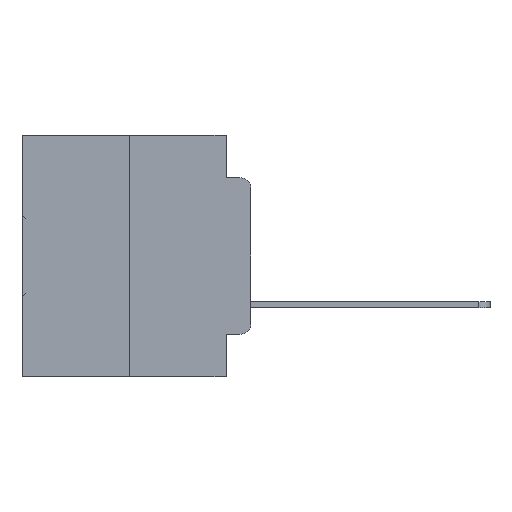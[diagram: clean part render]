
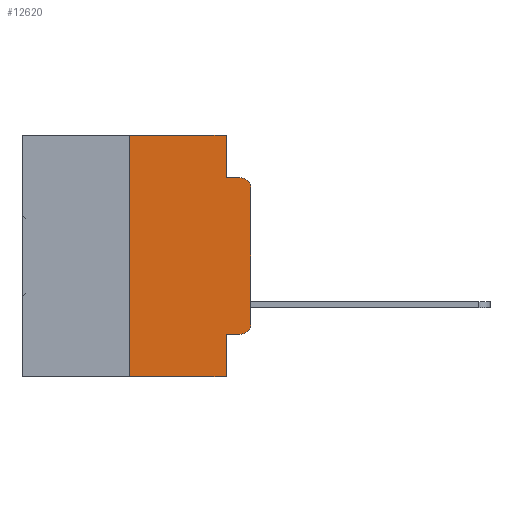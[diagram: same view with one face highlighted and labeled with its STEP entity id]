
A CAD part, left-side view. The second image highlights one B-rep face of the part: STEP entity #12620.
In plain terms, the highlighted planar face has unit normal (-1, 0, 0).
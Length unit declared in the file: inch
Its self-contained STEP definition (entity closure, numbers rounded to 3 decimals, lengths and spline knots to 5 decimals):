
#123 = AXIS2_PLACEMENT_3D ( 'NONE', #13753, #32018, #16451 ) ;
#330 = EDGE_CURVE ( 'NONE', #13568, #7716, #26120, .T. ) ;
#489 = ORIENTED_EDGE ( 'NONE', *, *, #15348, .F. ) ;
#678 = VERTEX_POINT ( 'NONE', #3235 ) ;
#837 = VECTOR ( 'NONE', #24182, 39.37008 ) ;
#2509 = VERTEX_POINT ( 'NONE', #14223 ) ;
#3235 = CARTESIAN_POINT ( 'NONE',  ( 0., 0.02, -0.0885 ) ) ;
#3309 = DIRECTION ( 'NONE',  ( 1., 0., 0. ) ) ;
#3755 = VECTOR ( 'NONE', #12663, 39.37008 ) ;
#3815 = DIRECTION ( 'NONE',  ( 0., 0., -1. ) ) ;
#3931 = CARTESIAN_POINT ( 'NONE',  ( 0., 0., -0.1085 ) ) ;
#4280 = CARTESIAN_POINT ( 'NONE',  ( 0., 0.051, -0.4115 ) ) ;
#6163 = VECTOR ( 'NONE', #3815, 39.37008 ) ;
#6385 = DIRECTION ( 'NONE',  ( 0., 0., -1. ) ) ;
#7286 = LINE ( 'NONE', #34816, #26885 ) ;
#7716 = VERTEX_POINT ( 'NONE', #9987 ) ;
#8122 = EDGE_CURVE ( 'NONE', #13568, #2509, #28965, .T. ) ;
#8532 = LINE ( 'NONE', #21666, #837 ) ;
#8862 = CIRCLE ( 'NONE', #123, 0.02 ) ;
#8866 = CARTESIAN_POINT ( 'NONE',  ( 0., 0.02, -0.1085 ) ) ;
#9408 = CARTESIAN_POINT ( 'NONE',  ( 0., 0.051, 0. ) ) ;
#9987 = CARTESIAN_POINT ( 'NONE',  ( 0., 0.02, -0.4115 ) ) ;
#10120 = VECTOR ( 'NONE', #23786, 39.37008 ) ;
#10635 = VECTOR ( 'NONE', #21236, 39.37008 ) ;
#10929 = ORIENTED_EDGE ( 'NONE', *, *, #330, .T. ) ;
#11174 = PLANE ( 'NONE',  #26160 ) ;
#11584 = DIRECTION ( 'NONE',  ( 0., 0., -1. ) ) ;
#11764 = EDGE_CURVE ( 'NONE', #28743, #16335, #8532, .T. ) ;
#12225 = CARTESIAN_POINT ( 'NONE',  ( 0., 0.051, 0. ) ) ;
#12292 = LINE ( 'NONE', #26441, #10635 ) ;
#12463 = EDGE_CURVE ( 'NONE', #16335, #32840, #12292, .T. ) ;
#12570 = VERTEX_POINT ( 'NONE', #13633 ) ;
#12620 = ADVANCED_FACE ( 'NONE', ( #28355 ), #11174, .F. ) ;
#12636 = CARTESIAN_POINT ( 'NONE',  ( 0., 0.25, 0. ) ) ;
#12663 = DIRECTION ( 'NONE',  ( 0., -1., 0. ) ) ;
#13158 = CIRCLE ( 'NONE', #15174, 0.02 ) ;
#13567 = EDGE_CURVE ( 'NONE', #32840, #33423, #14315, .T. ) ;
#13568 = VERTEX_POINT ( 'NONE', #28012 ) ;
#13633 = CARTESIAN_POINT ( 'NONE',  ( 0., 0., -0.3915 ) ) ;
#13753 = CARTESIAN_POINT ( 'NONE',  ( 0., 0.02, -0.3915 ) ) ;
#14223 = CARTESIAN_POINT ( 'NONE',  ( 0., 0.051, -0.5 ) ) ;
#14315 = LINE ( 'NONE', #12225, #6163 ) ;
#14411 = ORIENTED_EDGE ( 'NONE', *, *, #33435, .T. ) ;
#14981 = CARTESIAN_POINT ( 'NONE',  ( 0., 0.473, -0.5 ) ) ;
#15028 = VECTOR ( 'NONE', #6385, 39.37008 ) ;
#15174 = AXIS2_PLACEMENT_3D ( 'NONE', #8866, #27384, #11584 ) ;
#15348 = EDGE_CURVE ( 'NONE', #33423, #678, #7286, .T. ) ;
#16325 = CARTESIAN_POINT ( 'NONE',  ( 0., 0.051, -0.0885 ) ) ;
#16335 = VERTEX_POINT ( 'NONE', #12636 ) ;
#16451 = DIRECTION ( 'NONE',  ( 0., 0., -1. ) ) ;
#16666 = DIRECTION ( 'NONE',  ( 0., -1., 0. ) ) ;
#17501 = VERTEX_POINT ( 'NONE', #3931 ) ;
#17654 = LINE ( 'NONE', #14981, #30680 ) ;
#17664 = DIRECTION ( 'NONE',  ( 0., -1., 0. ) ) ;
#17928 = ORIENTED_EDGE ( 'NONE', *, *, #11764, .F. ) ;
#18853 = ORIENTED_EDGE ( 'NONE', *, *, #25952, .T. ) ;
#19766 = EDGE_LOOP ( 'NONE', ( #18853, #31314, #489, #32484, #20019, #17928, #33321, #31399, #10929, #14411 ) ) ;
#20019 = ORIENTED_EDGE ( 'NONE', *, *, #12463, .F. ) ;
#21179 = CARTESIAN_POINT ( 'NONE',  ( 0., 0., 0. ) ) ;
#21236 = DIRECTION ( 'NONE',  ( 0., -1., 0. ) ) ;
#21666 = CARTESIAN_POINT ( 'NONE',  ( 0., 0.25, 0. ) ) ;
#22361 = DIRECTION ( 'NONE',  ( 0., 0., -1. ) ) ;
#23786 = DIRECTION ( 'NONE',  ( 0., 0., 1. ) ) ;
#24182 = DIRECTION ( 'NONE',  ( 0., 0., 1. ) ) ;
#24256 = EDGE_CURVE ( 'NONE', #17501, #678, #13158, .T. ) ;
#25733 = EDGE_CURVE ( 'NONE', #28743, #2509, #17654, .T. ) ;
#25952 = EDGE_CURVE ( 'NONE', #12570, #17501, #31079, .T. ) ;
#26120 = LINE ( 'NONE', #4280, #3755 ) ;
#26160 = AXIS2_PLACEMENT_3D ( 'NONE', #29560, #3309, #22361 ) ;
#26441 = CARTESIAN_POINT ( 'NONE',  ( 0., 0.473, 0. ) ) ;
#26885 = VECTOR ( 'NONE', #16666, 39.37008 ) ;
#27384 = DIRECTION ( 'NONE',  ( -1., 0., 0. ) ) ;
#28012 = CARTESIAN_POINT ( 'NONE',  ( 0., 0.051, -0.4115 ) ) ;
#28355 = FACE_OUTER_BOUND ( 'NONE', #19766, .T. ) ;
#28743 = VERTEX_POINT ( 'NONE', #34099 ) ;
#28965 = LINE ( 'NONE', #32763, #15028 ) ;
#29560 = CARTESIAN_POINT ( 'NONE',  ( 0., 0.473, 0. ) ) ;
#30680 = VECTOR ( 'NONE', #17664, 39.37008 ) ;
#31079 = LINE ( 'NONE', #21179, #10120 ) ;
#31314 = ORIENTED_EDGE ( 'NONE', *, *, #24256, .T. ) ;
#31399 = ORIENTED_EDGE ( 'NONE', *, *, #8122, .F. ) ;
#32018 = DIRECTION ( 'NONE',  ( -1., 0., 0. ) ) ;
#32484 = ORIENTED_EDGE ( 'NONE', *, *, #13567, .F. ) ;
#32763 = CARTESIAN_POINT ( 'NONE',  ( 0., 0.051, 0. ) ) ;
#32840 = VERTEX_POINT ( 'NONE', #9408 ) ;
#33321 = ORIENTED_EDGE ( 'NONE', *, *, #25733, .T. ) ;
#33423 = VERTEX_POINT ( 'NONE', #16325 ) ;
#33435 = EDGE_CURVE ( 'NONE', #7716, #12570, #8862, .T. ) ;
#34099 = CARTESIAN_POINT ( 'NONE',  ( 0., 0.25, -0.5 ) ) ;
#34816 = CARTESIAN_POINT ( 'NONE',  ( 0., 0.051, -0.0885 ) ) ;
